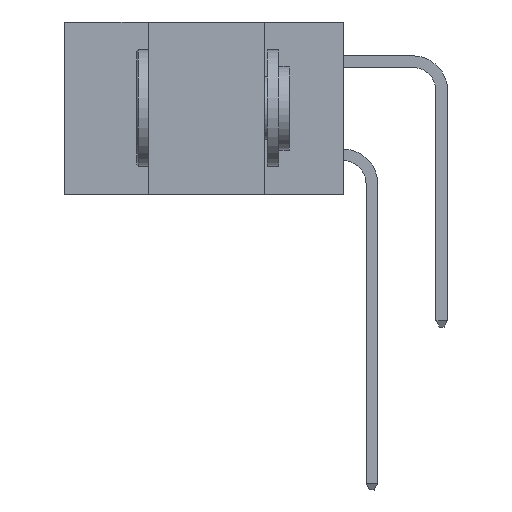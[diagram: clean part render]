
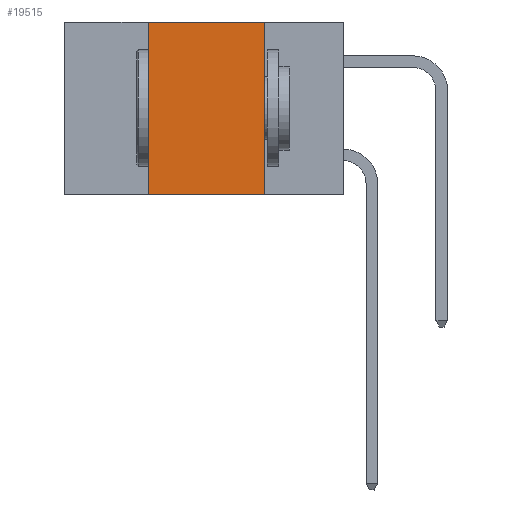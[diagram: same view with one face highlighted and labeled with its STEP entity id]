
A CAD part, left-side view. The second image highlights one B-rep face of the part: STEP entity #19515.
In plain terms, the highlighted planar face has unit normal (-1, 0, 0).
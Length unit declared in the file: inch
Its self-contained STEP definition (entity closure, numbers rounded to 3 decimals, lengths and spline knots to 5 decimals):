
#826 = FACE_OUTER_BOUND ( 'NONE', #26061, .T. ) ;
#1044 = VERTEX_POINT ( 'NONE', #17715 ) ;
#1580 = LINE ( 'NONE', #10889, #14659 ) ;
#3054 = CARTESIAN_POINT ( 'NONE',  ( 0., 0.42, 0. ) ) ;
#4597 = VERTEX_POINT ( 'NONE', #3054 ) ;
#5809 = ORIENTED_EDGE ( 'NONE', *, *, #11371, .T. ) ;
#8826 = DIRECTION ( 'NONE',  ( 0., 0., -1. ) ) ;
#8947 = DIRECTION ( 'NONE',  ( 0., -1., 0. ) ) ;
#10889 = CARTESIAN_POINT ( 'NONE',  ( 0., 0.6, 0. ) ) ;
#11371 = EDGE_CURVE ( 'NONE', #19348, #27057, #27141, .T. ) ;
#12350 = CARTESIAN_POINT ( 'NONE',  ( 0., 0.17, -0.37 ) ) ;
#13550 = LINE ( 'NONE', #27605, #29685 ) ;
#14031 = LINE ( 'NONE', #27922, #22155 ) ;
#14325 = VECTOR ( 'NONE', #8947, 39.37008 ) ;
#14584 = AXIS2_PLACEMENT_3D ( 'NONE', #21755, #24035, #14873 ) ;
#14659 = VECTOR ( 'NONE', #20212, 39.37008 ) ;
#14873 = DIRECTION ( 'NONE',  ( 0., 0., -1. ) ) ;
#17715 = CARTESIAN_POINT ( 'NONE',  ( 0., 0.17, 0. ) ) ;
#17963 = ORIENTED_EDGE ( 'NONE', *, *, #27008, .F. ) ;
#18677 = ORIENTED_EDGE ( 'NONE', *, *, #18888, .F. ) ;
#18888 = EDGE_CURVE ( 'NONE', #1044, #27057, #13550, .T. ) ;
#19287 = ORIENTED_EDGE ( 'NONE', *, *, #23315, .F. ) ;
#19316 = PLANE ( 'NONE',  #14584 ) ;
#19348 = VERTEX_POINT ( 'NONE', #27856 ) ;
#19515 = ADVANCED_FACE ( 'NONE', ( #826 ), #19316, .F. ) ;
#20212 = DIRECTION ( 'NONE',  ( 0., -1., 0. ) ) ;
#21755 = CARTESIAN_POINT ( 'NONE',  ( 0., 0.6, 0. ) ) ;
#22155 = VECTOR ( 'NONE', #30067, 39.37008 ) ;
#23315 = EDGE_CURVE ( 'NONE', #4597, #1044, #1580, .T. ) ;
#24035 = DIRECTION ( 'NONE',  ( 1., 0., 0. ) ) ;
#26061 = EDGE_LOOP ( 'NONE', ( #18677, #19287, #17963, #5809 ) ) ;
#27008 = EDGE_CURVE ( 'NONE', #19348, #4597, #14031, .T. ) ;
#27057 = VERTEX_POINT ( 'NONE', #12350 ) ;
#27141 = LINE ( 'NONE', #29420, #14325 ) ;
#27605 = CARTESIAN_POINT ( 'NONE',  ( 0., 0.17, -0.37 ) ) ;
#27856 = CARTESIAN_POINT ( 'NONE',  ( 0., 0.42, -0.37 ) ) ;
#27922 = CARTESIAN_POINT ( 'NONE',  ( 0., 0.42, -0.37 ) ) ;
#29420 = CARTESIAN_POINT ( 'NONE',  ( 0., 0.6, -0.37 ) ) ;
#29685 = VECTOR ( 'NONE', #8826, 39.37008 ) ;
#30067 = DIRECTION ( 'NONE',  ( 0., 0., 1. ) ) ;
